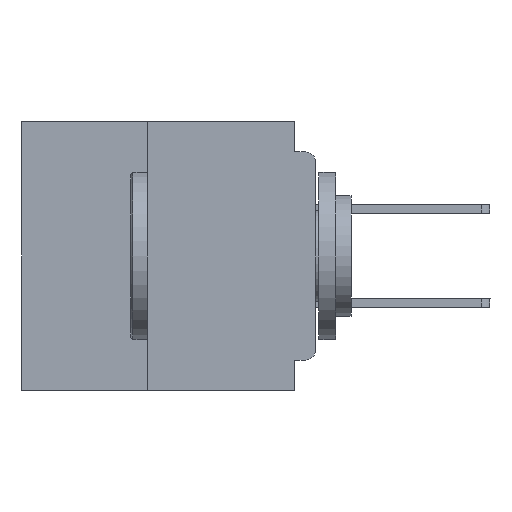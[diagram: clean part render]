
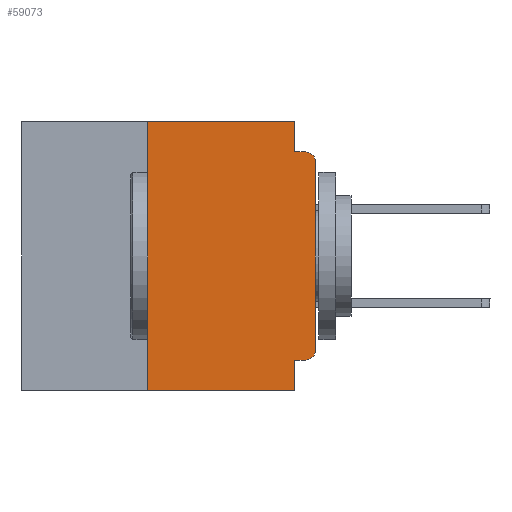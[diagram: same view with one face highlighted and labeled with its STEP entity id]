
A CAD part, left-side view. The second image highlights one B-rep face of the part: STEP entity #59073.
In plain terms, the highlighted planar face has unit normal (-1, 0, 0).
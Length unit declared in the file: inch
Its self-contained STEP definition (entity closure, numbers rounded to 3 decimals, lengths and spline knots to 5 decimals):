
#566 = DIRECTION ( 'NONE',  ( 0., 0., 1. ) ) ;
#1936 = CARTESIAN_POINT ( 'NONE',  ( 0., 0., -0.045 ) ) ;
#2092 = VERTEX_POINT ( 'NONE', #46390 ) ;
#2487 = EDGE_CURVE ( 'NONE', #37683, #13037, #56643, .T. ) ;
#2984 = ORIENTED_EDGE ( 'NONE', *, *, #7366, .T. ) ;
#5116 = DIRECTION ( 'NONE',  ( -1., 0., 0. ) ) ;
#5124 = CARTESIAN_POINT ( 'NONE',  ( 0., 0., 0. ) ) ;
#5668 = VERTEX_POINT ( 'NONE', #46095 ) ;
#5965 = ORIENTED_EDGE ( 'NONE', *, *, #49246, .T. ) ;
#7366 = EDGE_CURVE ( 'NONE', #46191, #25157, #52119, .T. ) ;
#9459 = EDGE_CURVE ( 'NONE', #25157, #37683, #18738, .T. ) ;
#10767 = ORIENTED_EDGE ( 'NONE', *, *, #36834, .F. ) ;
#10858 = CARTESIAN_POINT ( 'NONE',  ( 0., 0.031, -0.355 ) ) ;
#11669 = PLANE ( 'NONE',  #52524 ) ;
#12185 = FACE_OUTER_BOUND ( 'NONE', #41134, .T. ) ;
#12391 = CARTESIAN_POINT ( 'NONE',  ( 0., 0.031, 0. ) ) ;
#13037 = VERTEX_POINT ( 'NONE', #42600 ) ;
#13225 = VECTOR ( 'NONE', #566, 39.37008 ) ;
#13361 = DIRECTION ( 'NONE',  ( 0., -1., 0. ) ) ;
#14346 = DIRECTION ( 'NONE',  ( 0., 1., 0. ) ) ;
#16633 = DIRECTION ( 'NONE',  ( 1., 0., 0. ) ) ;
#18738 = LINE ( 'NONE', #5124, #57953 ) ;
#23020 = CARTESIAN_POINT ( 'NONE',  ( 0., 0.437, 0. ) ) ;
#24005 = VECTOR ( 'NONE', #27282, 39.37008 ) ;
#25005 = VERTEX_POINT ( 'NONE', #10858 ) ;
#25157 = VERTEX_POINT ( 'NONE', #31675 ) ;
#27282 = DIRECTION ( 'NONE',  ( 0., -1., 0. ) ) ;
#27454 = VECTOR ( 'NONE', #13361, 39.37008 ) ;
#28081 = CARTESIAN_POINT ( 'NONE',  ( 0., 0., -0.06 ) ) ;
#28942 = ORIENTED_EDGE ( 'NONE', *, *, #50050, .F. ) ;
#29016 = LINE ( 'NONE', #23020, #27454 ) ;
#29778 = VERTEX_POINT ( 'NONE', #37129 ) ;
#31019 = VECTOR ( 'NONE', #31411, 39.37008 ) ;
#31411 = DIRECTION ( 'NONE',  ( 0., -1., 0. ) ) ;
#31675 = CARTESIAN_POINT ( 'NONE',  ( 0., 0., -0.34 ) ) ;
#32707 = CARTESIAN_POINT ( 'NONE',  ( 0., 0.015, -0.355 ) ) ;
#32815 = CARTESIAN_POINT ( 'NONE',  ( 0., 0.031, -0.4 ) ) ;
#32890 = DIRECTION ( 'NONE',  ( 0., 0., -1. ) ) ;
#32951 = DIRECTION ( 'NONE',  ( -1., 0., 0. ) ) ;
#33023 = CARTESIAN_POINT ( 'NONE',  ( 0., 0.015, -0.06 ) ) ;
#34587 = CARTESIAN_POINT ( 'NONE',  ( 0., 0.015, -0.34 ) ) ;
#34594 = DIRECTION ( 'NONE',  ( 0., 0., 1. ) ) ;
#35019 = ORIENTED_EDGE ( 'NONE', *, *, #46231, .F. ) ;
#36834 = EDGE_CURVE ( 'NONE', #55390, #13037, #42583, .T. ) ;
#36995 = ORIENTED_EDGE ( 'NONE', *, *, #2487, .T. ) ;
#37129 = CARTESIAN_POINT ( 'NONE',  ( 0., 0.25, 0. ) ) ;
#37139 = LINE ( 'NONE', #46896, #24005 ) ;
#37312 = ORIENTED_EDGE ( 'NONE', *, *, #9459, .T. ) ;
#37683 = VERTEX_POINT ( 'NONE', #28081 ) ;
#39520 = EDGE_CURVE ( 'NONE', #2092, #55390, #61529, .T. ) ;
#39522 = DIRECTION ( 'NONE',  ( 0., 0., -1. ) ) ;
#40067 = VECTOR ( 'NONE', #14346, 39.37008 ) ;
#40930 = AXIS2_PLACEMENT_3D ( 'NONE', #33023, #32951, #32890 ) ;
#41134 = EDGE_LOOP ( 'NONE', ( #37312, #36995, #10767, #48121, #35019, #48546, #5965, #41739, #28942, #2984 ) ) ;
#41739 = ORIENTED_EDGE ( 'NONE', *, *, #53934, .F. ) ;
#41863 = DIRECTION ( 'NONE',  ( 0., 0., -1. ) ) ;
#42583 = LINE ( 'NONE', #1936, #31019 ) ;
#42600 = CARTESIAN_POINT ( 'NONE',  ( 0., 0.015, -0.045 ) ) ;
#44440 = AXIS2_PLACEMENT_3D ( 'NONE', #34587, #5116, #39522 ) ;
#44699 = CARTESIAN_POINT ( 'NONE',  ( 0., 0.25, -0.4 ) ) ;
#46095 = CARTESIAN_POINT ( 'NONE',  ( 0., 0.25, -0.4 ) ) ;
#46108 = CARTESIAN_POINT ( 'NONE',  ( 0., 0.437, 0. ) ) ;
#46191 = VERTEX_POINT ( 'NONE', #32707 ) ;
#46231 = EDGE_CURVE ( 'NONE', #29778, #2092, #29016, .T. ) ;
#46390 = CARTESIAN_POINT ( 'NONE',  ( 0., 0.031, 0. ) ) ;
#46896 = CARTESIAN_POINT ( 'NONE',  ( 0., 0.437, -0.4 ) ) ;
#48121 = ORIENTED_EDGE ( 'NONE', *, *, #39520, .F. ) ;
#48248 = VECTOR ( 'NONE', #57257, 39.37008 ) ;
#48498 = VECTOR ( 'NONE', #41863, 39.37008 ) ;
#48546 = ORIENTED_EDGE ( 'NONE', *, *, #56478, .F. ) ;
#49246 = EDGE_CURVE ( 'NONE', #5668, #52701, #37139, .T. ) ;
#50050 = EDGE_CURVE ( 'NONE', #46191, #25005, #53195, .T. ) ;
#51063 = DIRECTION ( 'NONE',  ( 0., 0., -1. ) ) ;
#52119 = CIRCLE ( 'NONE', #44440, 0.015 ) ;
#52333 = CARTESIAN_POINT ( 'NONE',  ( 0., 0.031, -0.4 ) ) ;
#52498 = LINE ( 'NONE', #44699, #13225 ) ;
#52524 = AXIS2_PLACEMENT_3D ( 'NONE', #46108, #16633, #51063 ) ;
#52701 = VERTEX_POINT ( 'NONE', #32815 ) ;
#53195 = LINE ( 'NONE', #58397, #40067 ) ;
#53934 = EDGE_CURVE ( 'NONE', #25005, #52701, #61278, .T. ) ;
#55390 = VERTEX_POINT ( 'NONE', #59237 ) ;
#56478 = EDGE_CURVE ( 'NONE', #5668, #29778, #52498, .T. ) ;
#56643 = CIRCLE ( 'NONE', #40930, 0.015 ) ;
#57257 = DIRECTION ( 'NONE',  ( 0., 0., -1. ) ) ;
#57953 = VECTOR ( 'NONE', #34594, 39.37008 ) ;
#58397 = CARTESIAN_POINT ( 'NONE',  ( 0., 0., -0.355 ) ) ;
#59073 = ADVANCED_FACE ( 'NONE', ( #12185 ), #11669, .F. ) ;
#59237 = CARTESIAN_POINT ( 'NONE',  ( 0., 0.031, -0.045 ) ) ;
#61278 = LINE ( 'NONE', #52333, #48248 ) ;
#61529 = LINE ( 'NONE', #12391, #48498 ) ;
